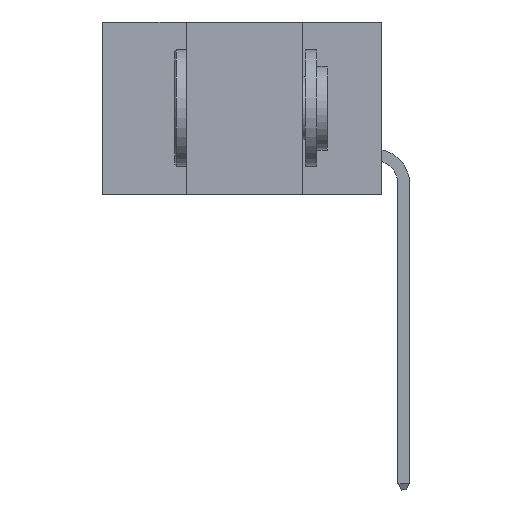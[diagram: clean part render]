
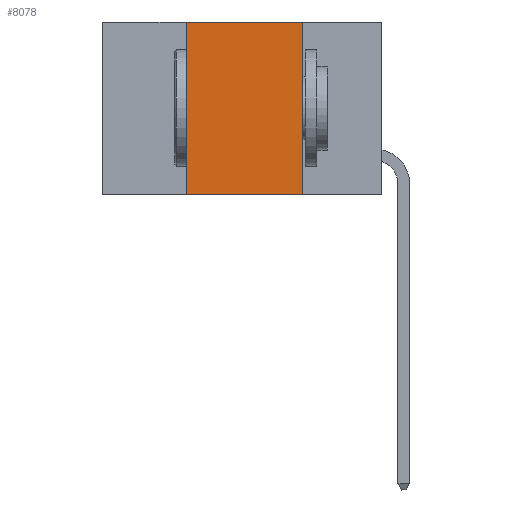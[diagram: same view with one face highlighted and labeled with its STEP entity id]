
A CAD part, left-side view. The second image highlights one B-rep face of the part: STEP entity #8078.
In plain terms, the highlighted planar face has unit normal (-1, 0, 0).
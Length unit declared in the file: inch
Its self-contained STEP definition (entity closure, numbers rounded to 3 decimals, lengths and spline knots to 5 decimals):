
#350 = PLANE ( 'NONE',  #19346 ) ;
#1872 = ORIENTED_EDGE ( 'NONE', *, *, #16506, .F. ) ;
#1906 = LINE ( 'NONE', #13738, #24870 ) ;
#2451 = DIRECTION ( 'NONE',  ( 1., 0., 0. ) ) ;
#2629 = VECTOR ( 'NONE', #20739, 39.37008 ) ;
#3555 = EDGE_LOOP ( 'NONE', ( #19443, #23208, #1872, #25397 ) ) ;
#3775 = DIRECTION ( 'NONE',  ( 0., -1., 0. ) ) ;
#4048 = EDGE_CURVE ( 'NONE', #5787, #24942, #17655, .T. ) ;
#4921 = VECTOR ( 'NONE', #17359, 39.37008 ) ;
#5787 = VERTEX_POINT ( 'NONE', #13611 ) ;
#5899 = CARTESIAN_POINT ( 'NONE',  ( 0., 0.17, 0. ) ) ;
#7607 = FACE_OUTER_BOUND ( 'NONE', #3555, .T. ) ;
#7761 = VERTEX_POINT ( 'NONE', #13946 ) ;
#8078 = ADVANCED_FACE ( 'NONE', ( #7607 ), #350, .F. ) ;
#8379 = VECTOR ( 'NONE', #3775, 39.37008 ) ;
#13611 = CARTESIAN_POINT ( 'NONE',  ( 0., 0.42, -0.37 ) ) ;
#13738 = CARTESIAN_POINT ( 'NONE',  ( 0., 0.42, 0. ) ) ;
#13873 = CARTESIAN_POINT ( 'NONE',  ( 0., 0.17, -0.37 ) ) ;
#13946 = CARTESIAN_POINT ( 'NONE',  ( 0., 0.42, 0. ) ) ;
#14649 = EDGE_CURVE ( 'NONE', #7761, #19513, #15456, .T. ) ;
#15381 = CARTESIAN_POINT ( 'NONE',  ( 0., 0.6, 0. ) ) ;
#15456 = LINE ( 'NONE', #15381, #4921 ) ;
#16259 = LINE ( 'NONE', #22826, #2629 ) ;
#16506 = EDGE_CURVE ( 'NONE', #5787, #7761, #1906, .T. ) ;
#17359 = DIRECTION ( 'NONE',  ( 0., -1., 0. ) ) ;
#17655 = LINE ( 'NONE', #25500, #8379 ) ;
#19346 = AXIS2_PLACEMENT_3D ( 'NONE', #22104, #2451, #22374 ) ;
#19443 = ORIENTED_EDGE ( 'NONE', *, *, #20776, .F. ) ;
#19513 = VERTEX_POINT ( 'NONE', #5899 ) ;
#20739 = DIRECTION ( 'NONE',  ( 0., 0., -1. ) ) ;
#20776 = EDGE_CURVE ( 'NONE', #19513, #24942, #16259, .T. ) ;
#22104 = CARTESIAN_POINT ( 'NONE',  ( 0., 0.6, 0. ) ) ;
#22374 = DIRECTION ( 'NONE',  ( 0., 0., -1. ) ) ;
#22826 = CARTESIAN_POINT ( 'NONE',  ( 0., 0.17, 0. ) ) ;
#23208 = ORIENTED_EDGE ( 'NONE', *, *, #14649, .F. ) ;
#24532 = DIRECTION ( 'NONE',  ( 0., 0., 1. ) ) ;
#24870 = VECTOR ( 'NONE', #24532, 39.37008 ) ;
#24942 = VERTEX_POINT ( 'NONE', #13873 ) ;
#25397 = ORIENTED_EDGE ( 'NONE', *, *, #4048, .T. ) ;
#25500 = CARTESIAN_POINT ( 'NONE',  ( 0., 0.6, -0.37 ) ) ;
